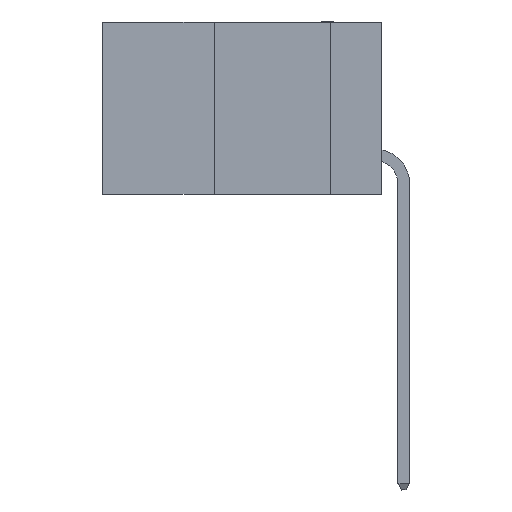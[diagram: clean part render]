
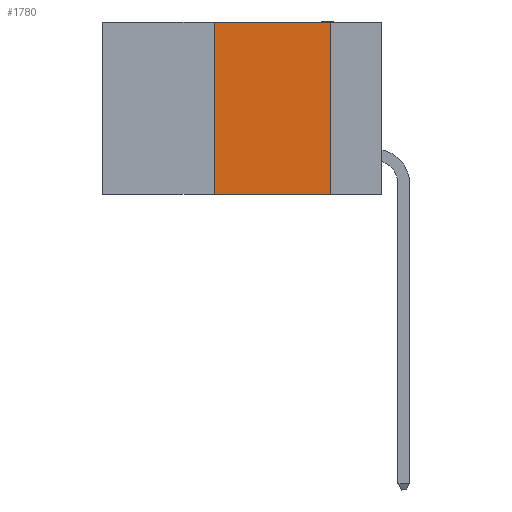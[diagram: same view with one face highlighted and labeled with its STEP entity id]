
A CAD part, left-side view. The second image highlights one B-rep face of the part: STEP entity #1780.
In plain terms, the highlighted planar face has unit normal (-1, 0, 0).
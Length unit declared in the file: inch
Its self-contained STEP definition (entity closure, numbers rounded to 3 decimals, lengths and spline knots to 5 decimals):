
#1780 = ADVANCED_FACE ( 'NONE', ( #20804 ), #24053, .F. ) ;
#2988 = DIRECTION ( 'NONE',  ( 0., -1., 0. ) ) ;
#4145 = DIRECTION ( 'NONE',  ( 0., 0., -1. ) ) ;
#6469 = DIRECTION ( 'NONE',  ( 1., 0., 0. ) ) ;
#7440 = LINE ( 'NONE', #20167, #24185 ) ;
#8913 = AXIS2_PLACEMENT_3D ( 'NONE', #25046, #6469, #25462 ) ;
#9572 = ORIENTED_EDGE ( 'NONE', *, *, #24884, .F. ) ;
#10177 = DIRECTION ( 'NONE',  ( 0., 0., 1. ) ) ;
#10818 = LINE ( 'NONE', #19137, #32469 ) ;
#13022 = CARTESIAN_POINT ( 'NONE',  ( 0., 0.36, 0. ) ) ;
#14044 = DIRECTION ( 'NONE',  ( 0., -1., 0. ) ) ;
#14049 = CARTESIAN_POINT ( 'NONE',  ( 0., 0.11, 0. ) ) ;
#15937 = EDGE_CURVE ( 'NONE', #35160, #29874, #7440, .T. ) ;
#18177 = LINE ( 'NONE', #13022, #19660 ) ;
#19137 = CARTESIAN_POINT ( 'NONE',  ( 0., 0.6, 0. ) ) ;
#19400 = VERTEX_POINT ( 'NONE', #23283 ) ;
#19660 = VECTOR ( 'NONE', #10177, 39.37008 ) ;
#20167 = CARTESIAN_POINT ( 'NONE',  ( 0., 0.6, -0.37 ) ) ;
#20804 = FACE_OUTER_BOUND ( 'NONE', #39016, .T. ) ;
#23036 = EDGE_CURVE ( 'NONE', #23129, #29874, #28002, .T. ) ;
#23129 = VERTEX_POINT ( 'NONE', #14049 ) ;
#23283 = CARTESIAN_POINT ( 'NONE',  ( 0., 0.36, 0. ) ) ;
#24053 = PLANE ( 'NONE',  #8913 ) ;
#24185 = VECTOR ( 'NONE', #14044, 39.37008 ) ;
#24884 = EDGE_CURVE ( 'NONE', #19400, #23129, #10818, .T. ) ;
#24966 = CARTESIAN_POINT ( 'NONE',  ( 0., 0.36, -0.37 ) ) ;
#25046 = CARTESIAN_POINT ( 'NONE',  ( 0., 0.6, 0. ) ) ;
#25462 = DIRECTION ( 'NONE',  ( 0., 0., -1. ) ) ;
#26992 = CARTESIAN_POINT ( 'NONE',  ( 0., 0.11, -0.37 ) ) ;
#27486 = ORIENTED_EDGE ( 'NONE', *, *, #35737, .F. ) ;
#28002 = LINE ( 'NONE', #33515, #37538 ) ;
#29032 = ORIENTED_EDGE ( 'NONE', *, *, #23036, .F. ) ;
#29874 = VERTEX_POINT ( 'NONE', #26992 ) ;
#32469 = VECTOR ( 'NONE', #2988, 39.37008 ) ;
#33515 = CARTESIAN_POINT ( 'NONE',  ( 0., 0.11, 0. ) ) ;
#35160 = VERTEX_POINT ( 'NONE', #24966 ) ;
#35737 = EDGE_CURVE ( 'NONE', #35160, #19400, #18177, .T. ) ;
#37538 = VECTOR ( 'NONE', #4145, 39.37008 ) ;
#39016 = EDGE_LOOP ( 'NONE', ( #29032, #9572, #27486, #41220 ) ) ;
#41220 = ORIENTED_EDGE ( 'NONE', *, *, #15937, .T. ) ;
